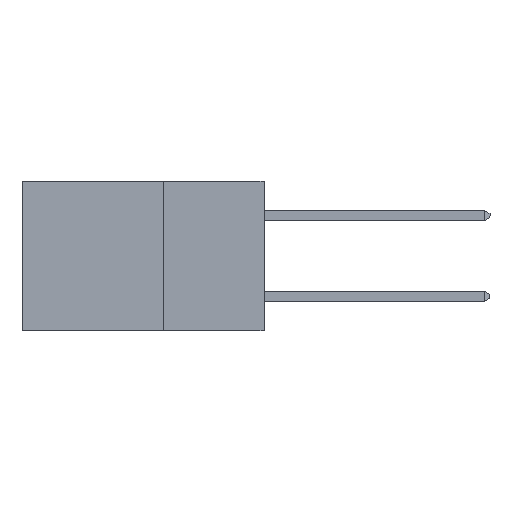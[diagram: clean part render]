
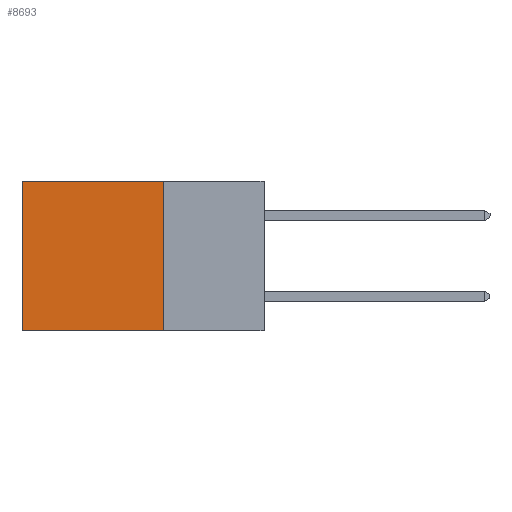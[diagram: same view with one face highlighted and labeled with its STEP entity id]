
A CAD part, left-side view. The second image highlights one B-rep face of the part: STEP entity #8693.
In plain terms, the highlighted planar face has unit normal (-1, 0, 0).
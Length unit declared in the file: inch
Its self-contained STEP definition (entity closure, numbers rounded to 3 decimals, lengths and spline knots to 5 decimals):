
#10 = DIRECTION ( 'NONE',  ( 0., 1., 0. ) ) ;
#791 = VECTOR ( 'NONE', #10, 39.37008 ) ;
#3548 = CARTESIAN_POINT ( 'NONE',  ( 0.298, 0.25, 0. ) ) ;
#3770 = DIRECTION ( 'NONE',  ( 0., 1., 0. ) ) ;
#4061 = CARTESIAN_POINT ( 'NONE',  ( 0.298, 0.25, 0. ) ) ;
#4766 = EDGE_LOOP ( 'NONE', ( #16679, #10302, #7544, #6377 ) ) ;
#4913 = CARTESIAN_POINT ( 'NONE',  ( 0.298, 0.25, -0.37 ) ) ;
#4962 = DIRECTION ( 'NONE',  ( 0., 0., -1. ) ) ;
#5058 = EDGE_CURVE ( 'NONE', #20764, #10966, #19320, .T. ) ;
#5360 = VERTEX_POINT ( 'NONE', #14953 ) ;
#5754 = DIRECTION ( 'NONE',  ( 0., 0., -1. ) ) ;
#6377 = ORIENTED_EDGE ( 'NONE', *, *, #6989, .T. ) ;
#6783 = CARTESIAN_POINT ( 'NONE',  ( 0.298, 0.25, -0.37 ) ) ;
#6989 = EDGE_CURVE ( 'NONE', #20764, #5360, #14631, .T. ) ;
#7544 = ORIENTED_EDGE ( 'NONE', *, *, #5058, .F. ) ;
#8452 = VERTEX_POINT ( 'NONE', #11607 ) ;
#8693 = ADVANCED_FACE ( 'NONE', ( #19504 ), #9063, .F. ) ;
#9063 = PLANE ( 'NONE',  #9276 ) ;
#9276 = AXIS2_PLACEMENT_3D ( 'NONE', #4061, #15744, #5754 ) ;
#10238 = VECTOR ( 'NONE', #3770, 39.37008 ) ;
#10302 = ORIENTED_EDGE ( 'NONE', *, *, #11611, .F. ) ;
#10966 = VERTEX_POINT ( 'NONE', #4913 ) ;
#11607 = CARTESIAN_POINT ( 'NONE',  ( 0.298, 0.6, -0.37 ) ) ;
#11611 = EDGE_CURVE ( 'NONE', #10966, #8452, #14151, .T. ) ;
#12784 = EDGE_CURVE ( 'NONE', #5360, #8452, #14129, .T. ) ;
#13319 = CARTESIAN_POINT ( 'NONE',  ( 0.298, 0.6, 0. ) ) ;
#13623 = VECTOR ( 'NONE', #4962, 39.37008 ) ;
#14129 = LINE ( 'NONE', #13319, #13623 ) ;
#14151 = LINE ( 'NONE', #6783, #791 ) ;
#14631 = LINE ( 'NONE', #3548, #10238 ) ;
#14865 = VECTOR ( 'NONE', #20947, 39.37008 ) ;
#14953 = CARTESIAN_POINT ( 'NONE',  ( 0.298, 0.6, 0. ) ) ;
#15744 = DIRECTION ( 'NONE',  ( 1., 0., 0. ) ) ;
#16679 = ORIENTED_EDGE ( 'NONE', *, *, #12784, .T. ) ;
#19320 = LINE ( 'NONE', #20583, #14865 ) ;
#19504 = FACE_OUTER_BOUND ( 'NONE', #4766, .T. ) ;
#20583 = CARTESIAN_POINT ( 'NONE',  ( 0.298, 0.25, 0. ) ) ;
#20676 = CARTESIAN_POINT ( 'NONE',  ( 0.298, 0.25, 0. ) ) ;
#20764 = VERTEX_POINT ( 'NONE', #20676 ) ;
#20947 = DIRECTION ( 'NONE',  ( 0., 0., -1. ) ) ;
